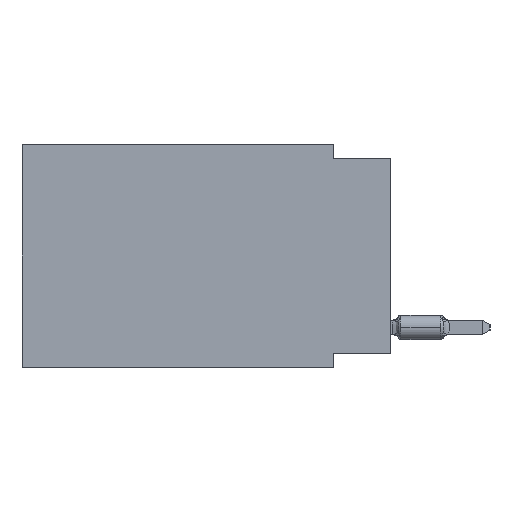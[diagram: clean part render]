
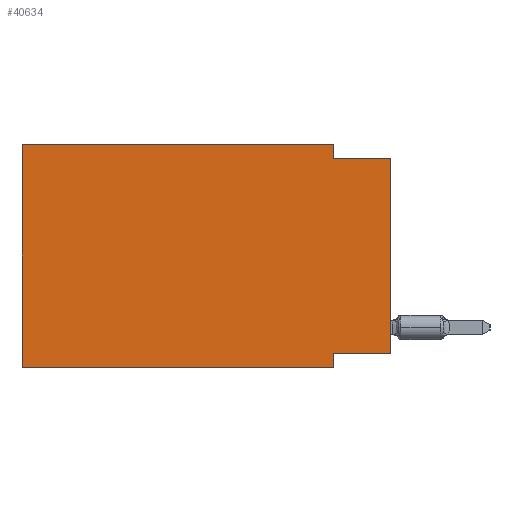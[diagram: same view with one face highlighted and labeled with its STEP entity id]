
A CAD part, left-side view. The second image highlights one B-rep face of the part: STEP entity #40634.
In plain terms, the highlighted planar face has unit normal (-1, 0, 0).
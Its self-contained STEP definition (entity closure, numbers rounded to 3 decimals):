
#170 = VERTEX_POINT ( 'NONE', #18032 ) ;
#1599 = DIRECTION ( 'NONE',  ( 0., -1., 0. ) ) ;
#2293 = LINE ( 'NONE', #45329, #56425 ) ;
#2702 = EDGE_CURVE ( 'NONE', #56513, #49720, #2293, .T. ) ;
#4423 = ORIENTED_EDGE ( 'NONE', *, *, #2702, .F. ) ;
#4486 = VECTOR ( 'NONE', #21347, 1000. ) ;
#5079 = DIRECTION ( 'NONE',  ( 0., 0., 1. ) ) ;
#5149 = ORIENTED_EDGE ( 'NONE', *, *, #57863, .F. ) ;
#6160 = ORIENTED_EDGE ( 'NONE', *, *, #6503, .T. ) ;
#6503 = EDGE_CURVE ( 'NONE', #56513, #23191, #17126, .T. ) ;
#7987 = VERTEX_POINT ( 'NONE', #35600 ) ;
#8324 = VECTOR ( 'NONE', #5079, 1000. ) ;
#9137 = CARTESIAN_POINT ( 'NONE',  ( 0., 2.54, -9.906 ) ) ;
#9486 = CARTESIAN_POINT ( 'NONE',  ( 0., 16.383, -9.906 ) ) ;
#9828 = DIRECTION ( 'NONE',  ( 0., -1., 0. ) ) ;
#12432 = CARTESIAN_POINT ( 'NONE',  ( 0., 2.54, 0. ) ) ;
#13652 = DIRECTION ( 'NONE',  ( 0., 1., 0. ) ) ;
#15642 = ORIENTED_EDGE ( 'NONE', *, *, #58487, .F. ) ;
#16736 = ORIENTED_EDGE ( 'NONE', *, *, #58008, .F. ) ;
#17126 = LINE ( 'NONE', #53781, #8324 ) ;
#18032 = CARTESIAN_POINT ( 'NONE',  ( 0., 2.54, -9.906 ) ) ;
#20743 = PLANE ( 'NONE',  #51811 ) ;
#21011 = LINE ( 'NONE', #37361, #4486 ) ;
#21090 = CARTESIAN_POINT ( 'NONE',  ( 0., 16.383, 0. ) ) ;
#21347 = DIRECTION ( 'NONE',  ( 0., -1., 0. ) ) ;
#23191 = VERTEX_POINT ( 'NONE', #52006 ) ;
#23970 = LINE ( 'NONE', #61292, #35956 ) ;
#24628 = VERTEX_POINT ( 'NONE', #28043 ) ;
#25854 = VERTEX_POINT ( 'NONE', #43255 ) ;
#27921 = CARTESIAN_POINT ( 'NONE',  ( 0., 2.54, -9.271 ) ) ;
#28043 = CARTESIAN_POINT ( 'NONE',  ( 0., 16.383, -9.906 ) ) ;
#32800 = VECTOR ( 'NONE', #9828, 1000. ) ;
#35196 = VECTOR ( 'NONE', #45812, 1000. ) ;
#35600 = CARTESIAN_POINT ( 'NONE',  ( 0., 16.383, 0. ) ) ;
#35956 = VECTOR ( 'NONE', #1599, 1000. ) ;
#37361 = CARTESIAN_POINT ( 'NONE',  ( 0., 16.383, 0. ) ) ;
#40634 = ADVANCED_FACE ( 'NONE', ( #53114 ), #20743, .F. ) ;
#41209 = EDGE_CURVE ( 'NONE', #25854, #23191, #23970, .T. ) ;
#43255 = CARTESIAN_POINT ( 'NONE',  ( 0., 2.54, -0.635 ) ) ;
#43885 = ORIENTED_EDGE ( 'NONE', *, *, #65335, .F. ) ;
#44477 = LINE ( 'NONE', #60088, #61216 ) ;
#44826 = DIRECTION ( 'NONE',  ( 0., 0., -1. ) ) ;
#45329 = CARTESIAN_POINT ( 'NONE',  ( 0., 0., -9.271 ) ) ;
#45812 = DIRECTION ( 'NONE',  ( 0., 0., -1. ) ) ;
#49720 = VERTEX_POINT ( 'NONE', #27921 ) ;
#49772 = EDGE_LOOP ( 'NONE', ( #6160, #58366, #43885, #5149, #16736, #55349, #15642, #4423 ) ) ;
#50142 = LINE ( 'NONE', #12432, #61488 ) ;
#51811 = AXIS2_PLACEMENT_3D ( 'NONE', #21090, #62712, #58098 ) ;
#52006 = CARTESIAN_POINT ( 'NONE',  ( 0., 0., -0.635 ) ) ;
#52890 = VERTEX_POINT ( 'NONE', #57201 ) ;
#53114 = FACE_OUTER_BOUND ( 'NONE', #49772, .T. ) ;
#53781 = CARTESIAN_POINT ( 'NONE',  ( 0., 0., 0. ) ) ;
#55349 = ORIENTED_EDGE ( 'NONE', *, *, #57506, .T. ) ;
#56425 = VECTOR ( 'NONE', #13652, 1000. ) ;
#56513 = VERTEX_POINT ( 'NONE', #56601 ) ;
#56601 = CARTESIAN_POINT ( 'NONE',  ( 0., 0., -9.271 ) ) ;
#57201 = CARTESIAN_POINT ( 'NONE',  ( 0., 2.54, 0. ) ) ;
#57506 = EDGE_CURVE ( 'NONE', #24628, #170, #58203, .T. ) ;
#57843 = LINE ( 'NONE', #9137, #35196 ) ;
#57863 = EDGE_CURVE ( 'NONE', #7987, #52890, #21011, .T. ) ;
#58008 = EDGE_CURVE ( 'NONE', #24628, #7987, #44477, .T. ) ;
#58098 = DIRECTION ( 'NONE',  ( 0., 0., -1. ) ) ;
#58203 = LINE ( 'NONE', #9486, #32800 ) ;
#58366 = ORIENTED_EDGE ( 'NONE', *, *, #41209, .F. ) ;
#58487 = EDGE_CURVE ( 'NONE', #49720, #170, #57843, .T. ) ;
#60088 = CARTESIAN_POINT ( 'NONE',  ( 0., 16.383, 0. ) ) ;
#61216 = VECTOR ( 'NONE', #66170, 1000. ) ;
#61292 = CARTESIAN_POINT ( 'NONE',  ( 0., 0., -0.635 ) ) ;
#61488 = VECTOR ( 'NONE', #44826, 1000. ) ;
#62712 = DIRECTION ( 'NONE',  ( 1., 0., 0. ) ) ;
#65335 = EDGE_CURVE ( 'NONE', #52890, #25854, #50142, .T. ) ;
#66170 = DIRECTION ( 'NONE',  ( 0., 0., 1. ) ) ;
